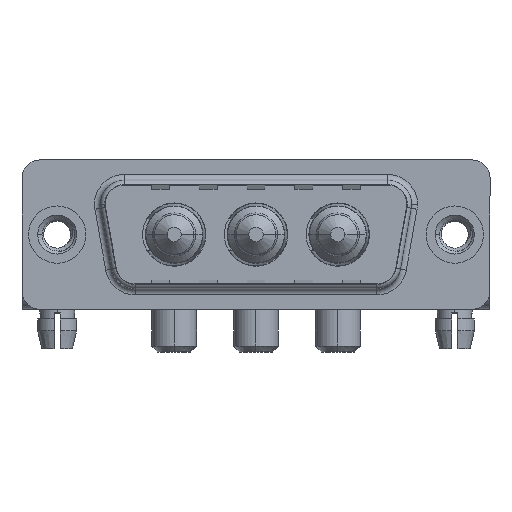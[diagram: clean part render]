
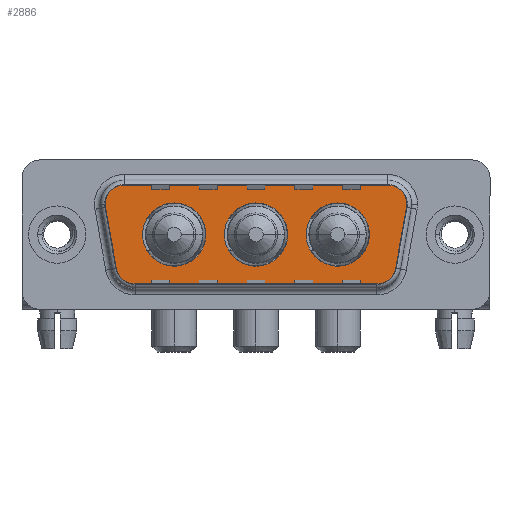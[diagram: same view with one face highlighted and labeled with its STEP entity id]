
A CAD part, top view. The second image highlights one B-rep face of the part: STEP entity #2886.
In plain terms, the highlighted planar face has unit normal (0, 0, 1).
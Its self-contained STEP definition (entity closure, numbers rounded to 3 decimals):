
#93 = VERTEX_POINT ( 'NONE', #12230 ) ;
#100 = ORIENTED_EDGE ( 'NONE', *, *, #12702, .T. ) ;
#116 = FACE_BOUND ( 'NONE', #9094, .T. ) ;
#187 = ORIENTED_EDGE ( 'NONE', *, *, #9448, .T. ) ;
#272 = CARTESIAN_POINT ( 'NONE',  ( 20.85, 0., 0. ) ) ;
#515 = VERTEX_POINT ( 'NONE', #11746 ) ;
#620 = CARTESIAN_POINT ( 'NONE',  ( 23.5, 0., 0. ) ) ;
#694 = AXIS2_PLACEMENT_3D ( 'NONE', #620, #9944, #14697 ) ;
#755 = VERTEX_POINT ( 'NONE', #12437 ) ;
#803 = VERTEX_POINT ( 'NONE', #12362 ) ;
#946 = CIRCLE ( 'NONE', #694, 2.65 ) ;
#1092 = DIRECTION ( 'NONE',  ( 0., 0., 1. ) ) ;
#1173 = VERTEX_POINT ( 'NONE', #272 ) ;
#1385 = CARTESIAN_POINT ( 'NONE',  ( 16.65, 0., 0. ) ) ;
#1572 = DIRECTION ( 'NONE',  ( 1., 0., 0. ) ) ;
#1675 = CIRCLE ( 'NONE', #10451, 2. ) ;
#1686 = DIRECTION ( 'NONE',  ( 0., 0., 1. ) ) ;
#1788 = VECTOR ( 'NONE', #13383, 1000. ) ;
#1820 = EDGE_LOOP ( 'NONE', ( #10864, #100, #11170, #13819, #14037, #4412, #6551, #187, #12363 ) ) ;
#1978 = EDGE_CURVE ( 'NONE', #1173, #803, #9039, .T. ) ;
#2003 = AXIS2_PLACEMENT_3D ( 'NONE', #8333, #13194, #2684 ) ;
#2033 = EDGE_CURVE ( 'NONE', #8985, #10474, #8599, .T. ) ;
#2182 = CARTESIAN_POINT ( 'NONE',  ( 29.859, 2.553, 0. ) ) ;
#2372 = AXIS2_PLACEMENT_3D ( 'NONE', #13617, #8759, #13459 ) ;
#2684 = DIRECTION ( 'NONE',  ( 1., 0., 0. ) ) ;
#2702 = CARTESIAN_POINT ( 'NONE',  ( 7.15, 0., 0. ) ) ;
#2815 = EDGE_CURVE ( 'NONE', #2893, #8985, #3259, .T. ) ;
#2886 = ADVANCED_FACE ( 'NONE', ( #10855, #116, #13340, #3701 ), #8482, .T. ) ;
#2893 = VERTEX_POINT ( 'NONE', #7387 ) ;
#2909 = EDGE_CURVE ( 'NONE', #2933, #2893, #13421, .T. ) ;
#2933 = VERTEX_POINT ( 'NONE', #13500 ) ;
#2952 = DIRECTION ( 'NONE',  ( 1., 0., 0. ) ) ;
#3070 = DIRECTION ( 'NONE',  ( 1., 0., 0. ) ) ;
#3182 = CARTESIAN_POINT ( 'NONE',  ( 6.434, -4.9, 0. ) ) ;
#3259 = CIRCLE ( 'NONE', #2003, 2. ) ;
#3697 = CIRCLE ( 'NONE', #12207, 2.65 ) ;
#3701 = FACE_OUTER_BOUND ( 'NONE', #1820, .T. ) ;
#3718 = VECTOR ( 'NONE', #2952, 1000. ) ;
#3779 = DIRECTION ( 'NONE',  ( 1., 0., 0. ) ) ;
#3922 = DIRECTION ( 'NONE',  ( 0., 0., 1. ) ) ;
#4087 = ORIENTED_EDGE ( 'NONE', *, *, #9180, .F. ) ;
#4412 = ORIENTED_EDGE ( 'NONE', *, *, #2815, .T. ) ;
#4427 = EDGE_CURVE ( 'NONE', #803, #1173, #946, .T. ) ;
#4804 = VERTEX_POINT ( 'NONE', #11813 ) ;
#4932 = EDGE_CURVE ( 'NONE', #5202, #4804, #14724, .T. ) ;
#5112 = VERTEX_POINT ( 'NONE', #15185 ) ;
#5122 = CARTESIAN_POINT ( 'NONE',  ( 27.889, 2.9, 0. ) ) ;
#5179 = DIRECTION ( 'NONE',  ( -1., 0., 0. ) ) ;
#5201 = DIRECTION ( 'NONE',  ( -1., 0., 0. ) ) ;
#5202 = VERTEX_POINT ( 'NONE', #7375 ) ;
#5585 = AXIS2_PLACEMENT_3D ( 'NONE', #9891, #3922, #3070 ) ;
#5675 = AXIS2_PLACEMENT_3D ( 'NONE', #5122, #1686, #5201 ) ;
#5745 = AXIS2_PLACEMENT_3D ( 'NONE', #9744, #14498, #3779 ) ;
#5860 = CIRCLE ( 'NONE', #2372, 2.65 ) ;
#6156 = DIRECTION ( 'NONE',  ( 1., 0., 0. ) ) ;
#6157 = DIRECTION ( 'NONE',  ( 0., 0., 1. ) ) ;
#6193 = VERTEX_POINT ( 'NONE', #2702 ) ;
#6211 = AXIS2_PLACEMENT_3D ( 'NONE', #12470, #9968, #1572 ) ;
#6350 = CARTESIAN_POINT ( 'NONE',  ( 5.411, 4.9, 0. ) ) ;
#6425 = AXIS2_PLACEMENT_3D ( 'NONE', #7904, #12689, #6790 ) ;
#6551 = ORIENTED_EDGE ( 'NONE', *, *, #2033, .T. ) ;
#6790 = DIRECTION ( 'NONE',  ( 1., 0., 0. ) ) ;
#7160 = CARTESIAN_POINT ( 'NONE',  ( 3.441, 2.553, 0. ) ) ;
#7375 = CARTESIAN_POINT ( 'NONE',  ( 29.859, 2.553, 0. ) ) ;
#7387 = CARTESIAN_POINT ( 'NONE',  ( 5.411, 4.9, 0. ) ) ;
#7516 = ORIENTED_EDGE ( 'NONE', *, *, #12612, .F. ) ;
#7570 = EDGE_LOOP ( 'NONE', ( #7516, #4087 ) ) ;
#7904 = CARTESIAN_POINT ( 'NONE',  ( 9.8, 0., 0. ) ) ;
#7938 = DIRECTION ( 'NONE',  ( 0., 0., 1. ) ) ;
#8029 = AXIS2_PLACEMENT_3D ( 'NONE', #8678, #12135, #6156 ) ;
#8101 = CIRCLE ( 'NONE', #5585, 2.65 ) ;
#8132 = LINE ( 'NONE', #2182, #9191 ) ;
#8198 = EDGE_CURVE ( 'NONE', #755, #12660, #5860, .T. ) ;
#8333 = CARTESIAN_POINT ( 'NONE',  ( 5.411, 2.9, 0. ) ) ;
#8482 = PLANE ( 'NONE',  #5745 ) ;
#8599 = LINE ( 'NONE', #11122, #1788 ) ;
#8607 = CARTESIAN_POINT ( 'NONE',  ( 6.434, -2.9, 0. ) ) ;
#8678 = CARTESIAN_POINT ( 'NONE',  ( 23.5, 0., 0. ) ) ;
#8759 = DIRECTION ( 'NONE',  ( 0., 0., 1. ) ) ;
#8985 = VERTEX_POINT ( 'NONE', #7160 ) ;
#9039 = CIRCLE ( 'NONE', #8029, 2.65 ) ;
#9085 = ORIENTED_EDGE ( 'NONE', *, *, #12892, .F. ) ;
#9094 = EDGE_LOOP ( 'NONE', ( #10790, #13376 ) ) ;
#9180 = EDGE_CURVE ( 'NONE', #6193, #515, #8101, .T. ) ;
#9191 = VECTOR ( 'NONE', #15393, 1000. ) ;
#9448 = EDGE_CURVE ( 'NONE', #10474, #93, #9872, .T. ) ;
#9744 = CARTESIAN_POINT ( 'NONE',  ( 26.866, -2.9, 0. ) ) ;
#9872 = CIRCLE ( 'NONE', #11882, 2. ) ;
#9891 = CARTESIAN_POINT ( 'NONE',  ( 9.8, 0., 0. ) ) ;
#9944 = DIRECTION ( 'NONE',  ( 0., 0., 1. ) ) ;
#9968 = DIRECTION ( 'NONE',  ( 0., 0., 1. ) ) ;
#10078 = ORIENTED_EDGE ( 'NONE', *, *, #8198, .F. ) ;
#10155 = CARTESIAN_POINT ( 'NONE',  ( 26.866, -4.9, 0. ) ) ;
#10314 = CARTESIAN_POINT ( 'NONE',  ( 27.889, 2.9, 0. ) ) ;
#10397 = LINE ( 'NONE', #3182, #3718 ) ;
#10451 = AXIS2_PLACEMENT_3D ( 'NONE', #10314, #7938, #12727 ) ;
#10474 = VERTEX_POINT ( 'NONE', #10775 ) ;
#10775 = CARTESIAN_POINT ( 'NONE',  ( 4.464, -3.247, 0. ) ) ;
#10790 = ORIENTED_EDGE ( 'NONE', *, *, #4427, .F. ) ;
#10855 = FACE_BOUND ( 'NONE', #12268, .T. ) ;
#10864 = ORIENTED_EDGE ( 'NONE', *, *, #14131, .T. ) ;
#11122 = CARTESIAN_POINT ( 'NONE',  ( 3.441, 2.553, 0. ) ) ;
#11170 = ORIENTED_EDGE ( 'NONE', *, *, #4932, .T. ) ;
#11710 = CIRCLE ( 'NONE', #6425, 2.65 ) ;
#11746 = CARTESIAN_POINT ( 'NONE',  ( 12.45, 0., 0. ) ) ;
#11813 = CARTESIAN_POINT ( 'NONE',  ( 29.889, 2.9, 0. ) ) ;
#11838 = DIRECTION ( 'NONE',  ( -1., 0., 0. ) ) ;
#11882 = AXIS2_PLACEMENT_3D ( 'NONE', #8607, #1092, #11838 ) ;
#12088 = VECTOR ( 'NONE', #5179, 1000. ) ;
#12135 = DIRECTION ( 'NONE',  ( 0., 0., 1. ) ) ;
#12207 = AXIS2_PLACEMENT_3D ( 'NONE', #1385, #6157, #14694 ) ;
#12230 = CARTESIAN_POINT ( 'NONE',  ( 6.434, -4.9, 0. ) ) ;
#12251 = EDGE_CURVE ( 'NONE', #4804, #2933, #1675, .T. ) ;
#12268 = EDGE_LOOP ( 'NONE', ( #9085, #10078 ) ) ;
#12362 = CARTESIAN_POINT ( 'NONE',  ( 26.15, 0., 0. ) ) ;
#12363 = ORIENTED_EDGE ( 'NONE', *, *, #15449, .T. ) ;
#12437 = CARTESIAN_POINT ( 'NONE',  ( 14., 0., 0. ) ) ;
#12470 = CARTESIAN_POINT ( 'NONE',  ( 26.866, -2.9, 0. ) ) ;
#12612 = EDGE_CURVE ( 'NONE', #515, #6193, #11710, .T. ) ;
#12660 = VERTEX_POINT ( 'NONE', #14002 ) ;
#12689 = DIRECTION ( 'NONE',  ( 0., 0., 1. ) ) ;
#12702 = EDGE_CURVE ( 'NONE', #5112, #5202, #8132, .T. ) ;
#12727 = DIRECTION ( 'NONE',  ( -1., 0., 0. ) ) ;
#12892 = EDGE_CURVE ( 'NONE', #12660, #755, #3697, .T. ) ;
#12990 = CIRCLE ( 'NONE', #6211, 2. ) ;
#13194 = DIRECTION ( 'NONE',  ( 0., 0., 1. ) ) ;
#13340 = FACE_BOUND ( 'NONE', #7570, .T. ) ;
#13376 = ORIENTED_EDGE ( 'NONE', *, *, #1978, .F. ) ;
#13383 = DIRECTION ( 'NONE',  ( 0.174, -0.985, 0. ) ) ;
#13421 = LINE ( 'NONE', #6350, #12088 ) ;
#13459 = DIRECTION ( 'NONE',  ( 1., 0., 0. ) ) ;
#13500 = CARTESIAN_POINT ( 'NONE',  ( 27.889, 4.9, 0. ) ) ;
#13617 = CARTESIAN_POINT ( 'NONE',  ( 16.65, 0., 0. ) ) ;
#13819 = ORIENTED_EDGE ( 'NONE', *, *, #12251, .T. ) ;
#14002 = CARTESIAN_POINT ( 'NONE',  ( 19.3, 0., 0. ) ) ;
#14037 = ORIENTED_EDGE ( 'NONE', *, *, #2909, .T. ) ;
#14131 = EDGE_CURVE ( 'NONE', #15367, #5112, #12990, .T. ) ;
#14498 = DIRECTION ( 'NONE',  ( 0., 0., 1. ) ) ;
#14694 = DIRECTION ( 'NONE',  ( 1., 0., 0. ) ) ;
#14697 = DIRECTION ( 'NONE',  ( 1., 0., 0. ) ) ;
#14724 = CIRCLE ( 'NONE', #5675, 2. ) ;
#15185 = CARTESIAN_POINT ( 'NONE',  ( 28.836, -3.247, 0. ) ) ;
#15367 = VERTEX_POINT ( 'NONE', #10155 ) ;
#15393 = DIRECTION ( 'NONE',  ( 0.174, 0.985, 0. ) ) ;
#15449 = EDGE_CURVE ( 'NONE', #93, #15367, #10397, .T. ) ;
